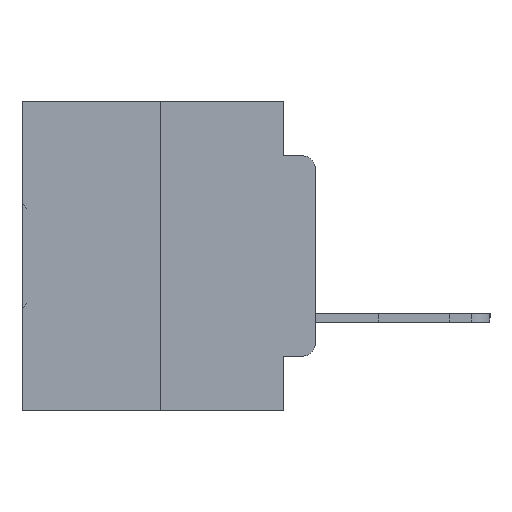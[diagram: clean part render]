
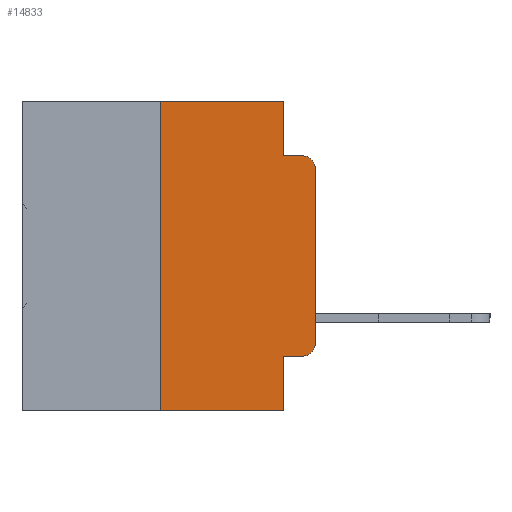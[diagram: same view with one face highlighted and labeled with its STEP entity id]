
A CAD part, left-side view. The second image highlights one B-rep face of the part: STEP entity #14833.
In plain terms, the highlighted planar face has unit normal (-1, 0, 0).
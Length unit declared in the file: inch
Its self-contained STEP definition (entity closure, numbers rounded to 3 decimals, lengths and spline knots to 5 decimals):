
#293 = LINE ( 'NONE', #1150, #14050 ) ;
#713 = ORIENTED_EDGE ( 'NONE', *, *, #15907, .F. ) ;
#722 = VECTOR ( 'NONE', #14738, 39.37008 ) ;
#1150 = CARTESIAN_POINT ( 'NONE',  ( 0., 0.473, -0.5 ) ) ;
#1517 = CARTESIAN_POINT ( 'NONE',  ( 0., 0., -0.3915 ) ) ;
#1773 = VERTEX_POINT ( 'NONE', #1517 ) ;
#4224 = ORIENTED_EDGE ( 'NONE', *, *, #19077, .T. ) ;
#4654 = ORIENTED_EDGE ( 'NONE', *, *, #10501, .F. ) ;
#4848 = FACE_OUTER_BOUND ( 'NONE', #22915, .T. ) ;
#4934 = CARTESIAN_POINT ( 'NONE',  ( 0., 0.25, 0. ) ) ;
#4969 = VERTEX_POINT ( 'NONE', #15750 ) ;
#6481 = CARTESIAN_POINT ( 'NONE',  ( 0., 0.051, -0.5 ) ) ;
#6613 = CARTESIAN_POINT ( 'NONE',  ( 0., 0.051, -0.0885 ) ) ;
#6878 = CIRCLE ( 'NONE', #21480, 0.02 ) ;
#7878 = CARTESIAN_POINT ( 'NONE',  ( 0., 0.051, -0.4115 ) ) ;
#8045 = EDGE_CURVE ( 'NONE', #20475, #29833, #9913, .T. ) ;
#8161 = CARTESIAN_POINT ( 'NONE',  ( 0., 0.051, 0. ) ) ;
#8225 = LINE ( 'NONE', #6613, #722 ) ;
#8672 = VECTOR ( 'NONE', #19493, 39.37008 ) ;
#9103 = VERTEX_POINT ( 'NONE', #19909 ) ;
#9528 = LINE ( 'NONE', #17049, #8672 ) ;
#9729 = AXIS2_PLACEMENT_3D ( 'NONE', #24811, #12448, #29701 ) ;
#9913 = LINE ( 'NONE', #4934, #27505 ) ;
#9958 = ORIENTED_EDGE ( 'NONE', *, *, #25613, .T. ) ;
#10374 = EDGE_CURVE ( 'NONE', #27621, #4969, #6878, .T. ) ;
#10501 = EDGE_CURVE ( 'NONE', #9103, #4969, #8225, .T. ) ;
#10688 = DIRECTION ( 'NONE',  ( 0., -1., 0. ) ) ;
#11104 = EDGE_CURVE ( 'NONE', #1773, #27621, #21707, .T. ) ;
#11704 = LINE ( 'NONE', #8161, #24139 ) ;
#11809 = LINE ( 'NONE', #20650, #30710 ) ;
#12298 = VERTEX_POINT ( 'NONE', #14776 ) ;
#12448 = DIRECTION ( 'NONE',  ( 1., 0., 0. ) ) ;
#14050 = VECTOR ( 'NONE', #17314, 39.37008 ) ;
#14075 = EDGE_CURVE ( 'NONE', #31386, #1773, #21184, .T. ) ;
#14082 = CARTESIAN_POINT ( 'NONE',  ( 0., 0.02, -0.1085 ) ) ;
#14245 = CARTESIAN_POINT ( 'NONE',  ( 0., 0.25, -0.5 ) ) ;
#14455 = CARTESIAN_POINT ( 'NONE',  ( 0., 0.02, -0.3915 ) ) ;
#14738 = DIRECTION ( 'NONE',  ( 0., -1., 0. ) ) ;
#14776 = CARTESIAN_POINT ( 'NONE',  ( 0., 0.051, -0.4115 ) ) ;
#14833 = ADVANCED_FACE ( 'NONE', ( #4848 ), #17405, .F. ) ;
#15214 = VECTOR ( 'NONE', #22835, 39.37008 ) ;
#15750 = CARTESIAN_POINT ( 'NONE',  ( 0., 0.02, -0.0885 ) ) ;
#15907 = EDGE_CURVE ( 'NONE', #29833, #16213, #11809, .T. ) ;
#16213 = VERTEX_POINT ( 'NONE', #19159 ) ;
#16571 = VERTEX_POINT ( 'NONE', #6481 ) ;
#16631 = DIRECTION ( 'NONE',  ( 0., 0., -1. ) ) ;
#16811 = ORIENTED_EDGE ( 'NONE', *, *, #32136, .F. ) ;
#16987 = DIRECTION ( 'NONE',  ( 0., 0., -1. ) ) ;
#17049 = CARTESIAN_POINT ( 'NONE',  ( 0., 0.051, 0. ) ) ;
#17314 = DIRECTION ( 'NONE',  ( 0., -1., 0. ) ) ;
#17405 = PLANE ( 'NONE',  #9729 ) ;
#17723 = LINE ( 'NONE', #7878, #23489 ) ;
#18331 = DIRECTION ( 'NONE',  ( 0., -1., 0. ) ) ;
#18353 = ORIENTED_EDGE ( 'NONE', *, *, #14075, .T. ) ;
#19077 = EDGE_CURVE ( 'NONE', #12298, #31386, #17723, .T. ) ;
#19159 = CARTESIAN_POINT ( 'NONE',  ( 0., 0.051, 0. ) ) ;
#19493 = DIRECTION ( 'NONE',  ( 0., 0., -1. ) ) ;
#19909 = CARTESIAN_POINT ( 'NONE',  ( 0., 0.051, -0.0885 ) ) ;
#20475 = VERTEX_POINT ( 'NONE', #14245 ) ;
#20575 = DIRECTION ( 'NONE',  ( 0., 0., 1. ) ) ;
#20650 = CARTESIAN_POINT ( 'NONE',  ( 0., 0.473, 0. ) ) ;
#21184 = CIRCLE ( 'NONE', #22761, 0.02 ) ;
#21480 = AXIS2_PLACEMENT_3D ( 'NONE', #14082, #31235, #16631 ) ;
#21707 = LINE ( 'NONE', #32513, #15214 ) ;
#21714 = EDGE_CURVE ( 'NONE', #16213, #9103, #11704, .T. ) ;
#21750 = ORIENTED_EDGE ( 'NONE', *, *, #8045, .F. ) ;
#22761 = AXIS2_PLACEMENT_3D ( 'NONE', #14455, #31589, #16987 ) ;
#22835 = DIRECTION ( 'NONE',  ( 0., 0., 1. ) ) ;
#22915 = EDGE_LOOP ( 'NONE', ( #23704, #24472, #4654, #32414, #713, #21750, #9958, #16811, #4224, #18353 ) ) ;
#23489 = VECTOR ( 'NONE', #18331, 39.37008 ) ;
#23704 = ORIENTED_EDGE ( 'NONE', *, *, #11104, .T. ) ;
#24139 = VECTOR ( 'NONE', #33115, 39.37008 ) ;
#24472 = ORIENTED_EDGE ( 'NONE', *, *, #10374, .T. ) ;
#24811 = CARTESIAN_POINT ( 'NONE',  ( 0., 0.473, 0. ) ) ;
#25613 = EDGE_CURVE ( 'NONE', #20475, #16571, #293, .T. ) ;
#27505 = VECTOR ( 'NONE', #20575, 39.37008 ) ;
#27542 = CARTESIAN_POINT ( 'NONE',  ( 0., 0., -0.1085 ) ) ;
#27621 = VERTEX_POINT ( 'NONE', #27542 ) ;
#28395 = CARTESIAN_POINT ( 'NONE',  ( 0., 0.25, 0. ) ) ;
#29701 = DIRECTION ( 'NONE',  ( 0., 0., -1. ) ) ;
#29833 = VERTEX_POINT ( 'NONE', #28395 ) ;
#30710 = VECTOR ( 'NONE', #10688, 39.37008 ) ;
#31235 = DIRECTION ( 'NONE',  ( -1., 0., 0. ) ) ;
#31386 = VERTEX_POINT ( 'NONE', #31891 ) ;
#31589 = DIRECTION ( 'NONE',  ( -1., 0., 0. ) ) ;
#31891 = CARTESIAN_POINT ( 'NONE',  ( 0., 0.02, -0.4115 ) ) ;
#32136 = EDGE_CURVE ( 'NONE', #12298, #16571, #9528, .T. ) ;
#32414 = ORIENTED_EDGE ( 'NONE', *, *, #21714, .F. ) ;
#32513 = CARTESIAN_POINT ( 'NONE',  ( 0., 0., 0. ) ) ;
#33115 = DIRECTION ( 'NONE',  ( 0., 0., -1. ) ) ;
